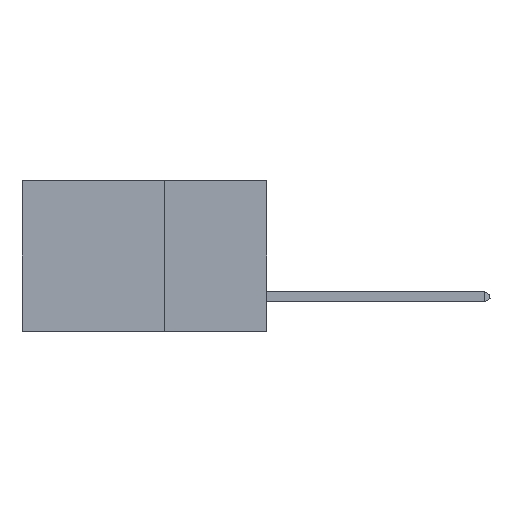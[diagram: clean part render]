
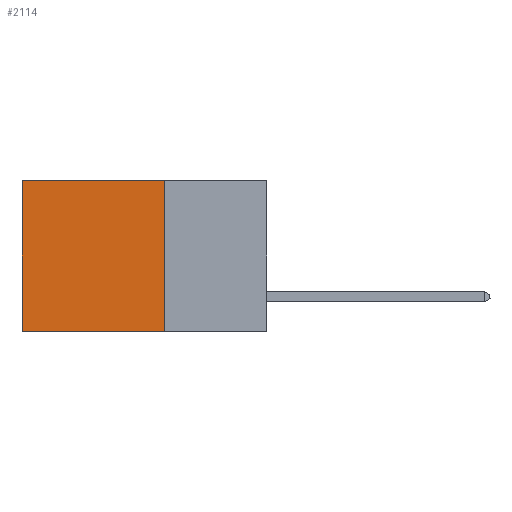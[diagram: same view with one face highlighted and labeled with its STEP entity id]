
A CAD part, left-side view. The second image highlights one B-rep face of the part: STEP entity #2114.
In plain terms, the highlighted planar face has unit normal (-1, 0, 0).
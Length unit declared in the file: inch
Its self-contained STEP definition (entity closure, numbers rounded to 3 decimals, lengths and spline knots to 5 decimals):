
#213 = EDGE_LOOP ( 'NONE', ( #13097, #12908, #20481, #22668 ) ) ;
#1248 = LINE ( 'NONE', #18631, #9184 ) ;
#2053 = VECTOR ( 'NONE', #8193, 39.37008 ) ;
#2114 = ADVANCED_FACE ( 'NONE', ( #5619 ), #20077, .F. ) ;
#2883 = CARTESIAN_POINT ( 'NONE',  ( 0.2875, 0.6, 0. ) ) ;
#3032 = CARTESIAN_POINT ( 'NONE',  ( 0.2875, 0.6, -0.37 ) ) ;
#3817 = LINE ( 'NONE', #16064, #17768 ) ;
#3922 = LINE ( 'NONE', #12789, #19543 ) ;
#4766 = AXIS2_PLACEMENT_3D ( 'NONE', #11116, #5468, #20226 ) ;
#5364 = EDGE_CURVE ( 'NONE', #20961, #19274, #3922, .T. ) ;
#5468 = DIRECTION ( 'NONE',  ( 1., 0., 0. ) ) ;
#5619 = FACE_OUTER_BOUND ( 'NONE', #213, .T. ) ;
#5823 = VERTEX_POINT ( 'NONE', #3032 ) ;
#8193 = DIRECTION ( 'NONE',  ( 0., 1., 0. ) ) ;
#9153 = LINE ( 'NONE', #17405, #2053 ) ;
#9184 = VECTOR ( 'NONE', #22758, 39.37008 ) ;
#10102 = CARTESIAN_POINT ( 'NONE',  ( 0.2875, 0.25, -0.37 ) ) ;
#10880 = DIRECTION ( 'NONE',  ( 0., 1., 0. ) ) ;
#11116 = CARTESIAN_POINT ( 'NONE',  ( 0.2875, 0.25, 0. ) ) ;
#12789 = CARTESIAN_POINT ( 'NONE',  ( 0.2875, 0.25, 0. ) ) ;
#12908 = ORIENTED_EDGE ( 'NONE', *, *, #20493, .F. ) ;
#13097 = ORIENTED_EDGE ( 'NONE', *, *, #14495, .T. ) ;
#13514 = VERTEX_POINT ( 'NONE', #2883 ) ;
#14495 = EDGE_CURVE ( 'NONE', #13514, #5823, #1248, .T. ) ;
#16064 = CARTESIAN_POINT ( 'NONE',  ( 0.2875, 0.25, -0.37 ) ) ;
#16189 = DIRECTION ( 'NONE',  ( 0., 0., -1. ) ) ;
#17405 = CARTESIAN_POINT ( 'NONE',  ( 0.2875, 0.25, 0. ) ) ;
#17768 = VECTOR ( 'NONE', #10880, 39.37008 ) ;
#18631 = CARTESIAN_POINT ( 'NONE',  ( 0.2875, 0.6, 0. ) ) ;
#19274 = VERTEX_POINT ( 'NONE', #10102 ) ;
#19543 = VECTOR ( 'NONE', #16189, 39.37008 ) ;
#20077 = PLANE ( 'NONE',  #4766 ) ;
#20226 = DIRECTION ( 'NONE',  ( 0., 0., -1. ) ) ;
#20481 = ORIENTED_EDGE ( 'NONE', *, *, #5364, .F. ) ;
#20493 = EDGE_CURVE ( 'NONE', #19274, #5823, #3817, .T. ) ;
#20961 = VERTEX_POINT ( 'NONE', #22624 ) ;
#22338 = EDGE_CURVE ( 'NONE', #20961, #13514, #9153, .T. ) ;
#22624 = CARTESIAN_POINT ( 'NONE',  ( 0.2875, 0.25, 0. ) ) ;
#22668 = ORIENTED_EDGE ( 'NONE', *, *, #22338, .T. ) ;
#22758 = DIRECTION ( 'NONE',  ( 0., 0., -1. ) ) ;
